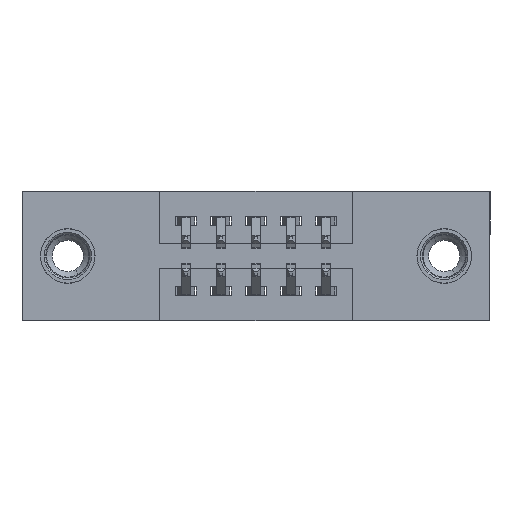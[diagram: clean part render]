
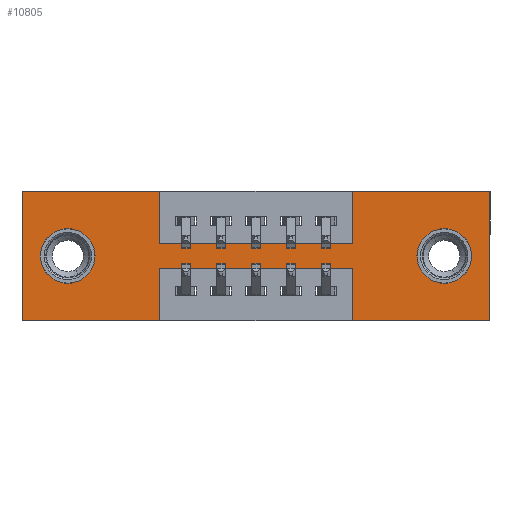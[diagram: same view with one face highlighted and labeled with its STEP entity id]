
A CAD part, front view. The second image highlights one B-rep face of the part: STEP entity #10805.
In plain terms, the highlighted planar face has unit normal (0, -1, 0).
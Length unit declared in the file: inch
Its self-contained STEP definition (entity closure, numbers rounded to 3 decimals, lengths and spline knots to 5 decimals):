
#29 = VERTEX_POINT ( 'NONE', #152 ) ;
#90 = LINE ( 'NONE', #10224, #9237 ) ;
#152 = CARTESIAN_POINT ( 'NONE',  ( 0.3925, 0., -0.37 ) ) ;
#196 = LINE ( 'NONE', #558, #7060 ) ;
#227 = DIRECTION ( 'NONE',  ( 0., -1., 0. ) ) ;
#324 = CARTESIAN_POINT ( 'NONE',  ( 0.9425, 0., -0.37 ) ) ;
#452 = DIRECTION ( 'NONE',  ( 0., 1., 0. ) ) ;
#520 = EDGE_LOOP ( 'NONE', ( #9153, #6924 ) ) ;
#558 = CARTESIAN_POINT ( 'NONE',  ( 0., 0., 0. ) ) ;
#603 = CARTESIAN_POINT ( 'NONE',  ( 0.13, 0., -0.107 ) ) ;
#827 = VERTEX_POINT ( 'NONE', #324 ) ;
#832 = EDGE_LOOP ( 'NONE', ( #2418, #1448 ) ) ;
#889 = CARTESIAN_POINT ( 'NONE',  ( 0.3925, 0., 0. ) ) ;
#953 = VERTEX_POINT ( 'NONE', #5917 ) ;
#1005 = AXIS2_PLACEMENT_3D ( 'NONE', #3215, #3204, #3176 ) ;
#1339 = CARTESIAN_POINT ( 'NONE',  ( 1.205, 0., -0.263 ) ) ;
#1391 = EDGE_CURVE ( 'NONE', #9028, #10332, #6580, .T. ) ;
#1403 = CARTESIAN_POINT ( 'NONE',  ( 0.9425, 0., -0.22 ) ) ;
#1415 = LINE ( 'NONE', #2271, #8147 ) ;
#1448 = ORIENTED_EDGE ( 'NONE', *, *, #3279, .T. ) ;
#1508 = ORIENTED_EDGE ( 'NONE', *, *, #8458, .F. ) ;
#1509 = DIRECTION ( 'NONE',  ( 1., 0., 0. ) ) ;
#1518 = ORIENTED_EDGE ( 'NONE', *, *, #10846, .F. ) ;
#1532 = VERTEX_POINT ( 'NONE', #1730 ) ;
#1537 = ORIENTED_EDGE ( 'NONE', *, *, #2017, .F. ) ;
#1550 = ORIENTED_EDGE ( 'NONE', *, *, #4668, .F. ) ;
#1585 = VECTOR ( 'NONE', #7772, 39.37008 ) ;
#1627 = EDGE_CURVE ( 'NONE', #7765, #827, #2035, .T. ) ;
#1730 = CARTESIAN_POINT ( 'NONE',  ( 0.9425, 0., -0.15 ) ) ;
#1786 = VERTEX_POINT ( 'NONE', #5215 ) ;
#1907 = EDGE_CURVE ( 'NONE', #4966, #5875, #4269, .T. ) ;
#2017 = EDGE_CURVE ( 'NONE', #3804, #7765, #5491, .T. ) ;
#2035 = LINE ( 'NONE', #3509, #6430 ) ;
#2183 = DIRECTION ( 'NONE',  ( 0., 0., 1. ) ) ;
#2238 = VECTOR ( 'NONE', #8586, 39.37008 ) ;
#2268 = CARTESIAN_POINT ( 'NONE',  ( 0.3925, 0., -0.22 ) ) ;
#2271 = CARTESIAN_POINT ( 'NONE',  ( 0.9425, 0., -0.37 ) ) ;
#2400 = EDGE_CURVE ( 'NONE', #10332, #29, #6279, .T. ) ;
#2418 = ORIENTED_EDGE ( 'NONE', *, *, #10934, .T. ) ;
#2457 = LINE ( 'NONE', #4250, #9087 ) ;
#2531 = EDGE_CURVE ( 'NONE', #4378, #1532, #5475, .T. ) ;
#2678 = CARTESIAN_POINT ( 'NONE',  ( 0.13, 0., -0.185 ) ) ;
#3044 = CARTESIAN_POINT ( 'NONE',  ( 0.9425, 0., 0. ) ) ;
#3176 = DIRECTION ( 'NONE',  ( 0., 0., 1. ) ) ;
#3204 = DIRECTION ( 'NONE',  ( 0., 1., 0. ) ) ;
#3215 = CARTESIAN_POINT ( 'NONE',  ( 0.13, 0., -0.185 ) ) ;
#3248 = LINE ( 'NONE', #9326, #9822 ) ;
#3279 = EDGE_CURVE ( 'NONE', #10318, #953, #9589, .T. ) ;
#3509 = CARTESIAN_POINT ( 'NONE',  ( 0., 0., -0.37 ) ) ;
#3572 = DIRECTION ( 'NONE',  ( 0., 0., 1. ) ) ;
#3727 = DIRECTION ( 'NONE',  ( 0., 0., -1. ) ) ;
#3750 = DIRECTION ( 'NONE',  ( 0., 1., 0. ) ) ;
#3784 = CARTESIAN_POINT ( 'NONE',  ( 1.205, 0., -0.185 ) ) ;
#3804 = VERTEX_POINT ( 'NONE', #10562 ) ;
#3896 = EDGE_CURVE ( 'NONE', #29, #6833, #3248, .T. ) ;
#3912 = CARTESIAN_POINT ( 'NONE',  ( 0., 0., -0.37 ) ) ;
#4129 = EDGE_CURVE ( 'NONE', #5875, #4966, #5434, .T. ) ;
#4250 = CARTESIAN_POINT ( 'NONE',  ( 0., 0., 0. ) ) ;
#4269 = CIRCLE ( 'NONE', #1005, 0.078 ) ;
#4378 = VERTEX_POINT ( 'NONE', #5546 ) ;
#4589 = LINE ( 'NONE', #7727, #2238 ) ;
#4656 = CARTESIAN_POINT ( 'NONE',  ( 0.13, 0., -0.263 ) ) ;
#4668 = EDGE_CURVE ( 'NONE', #1786, #3804, #4589, .T. ) ;
#4685 = ORIENTED_EDGE ( 'NONE', *, *, #9633, .F. ) ;
#4820 = CARTESIAN_POINT ( 'NONE',  ( 0., 0., -0.37 ) ) ;
#4946 = VECTOR ( 'NONE', #2183, 39.37008 ) ;
#4947 = DIRECTION ( 'NONE',  ( 0., 0., 1. ) ) ;
#4966 = VERTEX_POINT ( 'NONE', #4656 ) ;
#5127 = DIRECTION ( 'NONE',  ( 0., 0., -1. ) ) ;
#5215 = CARTESIAN_POINT ( 'NONE',  ( 0.9425, 0., 0. ) ) ;
#5327 = DIRECTION ( 'NONE',  ( -1., 0., 0. ) ) ;
#5373 = ORIENTED_EDGE ( 'NONE', *, *, #1391, .F. ) ;
#5434 = CIRCLE ( 'NONE', #10303, 0.078 ) ;
#5475 = LINE ( 'NONE', #7199, #9731 ) ;
#5491 = LINE ( 'NONE', #5619, #9745 ) ;
#5495 = FACE_BOUND ( 'NONE', #832, .T. ) ;
#5546 = CARTESIAN_POINT ( 'NONE',  ( 0.3925, 0., -0.15 ) ) ;
#5549 = DIRECTION ( 'NONE',  ( 0., 0., -1. ) ) ;
#5619 = CARTESIAN_POINT ( 'NONE',  ( 1.335, 0., 0. ) ) ;
#5656 = PLANE ( 'NONE',  #7951 ) ;
#5764 = FACE_BOUND ( 'NONE', #520, .T. ) ;
#5801 = ORIENTED_EDGE ( 'NONE', *, *, #3896, .F. ) ;
#5832 = CARTESIAN_POINT ( 'NONE',  ( 1.205, 0., -0.185 ) ) ;
#5875 = VERTEX_POINT ( 'NONE', #603 ) ;
#5917 = CARTESIAN_POINT ( 'NONE',  ( 1.205, 0., -0.107 ) ) ;
#5991 = CARTESIAN_POINT ( 'NONE',  ( 0.3925, 0., -0.37 ) ) ;
#6013 = ORIENTED_EDGE ( 'NONE', *, *, #2531, .F. ) ;
#6158 = CIRCLE ( 'NONE', #10194, 0.078 ) ;
#6216 = ORIENTED_EDGE ( 'NONE', *, *, #2400, .F. ) ;
#6279 = LINE ( 'NONE', #5991, #1585 ) ;
#6430 = VECTOR ( 'NONE', #5327, 39.37008 ) ;
#6432 = ORIENTED_EDGE ( 'NONE', *, *, #9747, .F. ) ;
#6515 = DIRECTION ( 'NONE',  ( 0., 0., -1. ) ) ;
#6580 = LINE ( 'NONE', #8602, #10785 ) ;
#6704 = DIRECTION ( 'NONE',  ( 0., 0., -1. ) ) ;
#6833 = VERTEX_POINT ( 'NONE', #4820 ) ;
#6924 = ORIENTED_EDGE ( 'NONE', *, *, #1907, .T. ) ;
#7060 = VECTOR ( 'NONE', #1509, 39.37008 ) ;
#7199 = CARTESIAN_POINT ( 'NONE',  ( 0.3925, 0., -0.15 ) ) ;
#7727 = CARTESIAN_POINT ( 'NONE',  ( 0., 0., 0. ) ) ;
#7765 = VERTEX_POINT ( 'NONE', #10062 ) ;
#7772 = DIRECTION ( 'NONE',  ( 0., 0., -1. ) ) ;
#7951 = AXIS2_PLACEMENT_3D ( 'NONE', #3912, #227, #6515 ) ;
#8147 = VECTOR ( 'NONE', #4947, 39.37008 ) ;
#8458 = EDGE_CURVE ( 'NONE', #6833, #10742, #2457, .T. ) ;
#8586 = DIRECTION ( 'NONE',  ( 1., 0., 0. ) ) ;
#8602 = CARTESIAN_POINT ( 'NONE',  ( 0.3925, 0., -0.22 ) ) ;
#8731 = DIRECTION ( 'NONE',  ( 0., 1., 0. ) ) ;
#9028 = VERTEX_POINT ( 'NONE', #1403 ) ;
#9087 = VECTOR ( 'NONE', #10974, 39.37008 ) ;
#9130 = ORIENTED_EDGE ( 'NONE', *, *, #10443, .F. ) ;
#9153 = ORIENTED_EDGE ( 'NONE', *, *, #4129, .T. ) ;
#9237 = VECTOR ( 'NONE', #5127, 39.37008 ) ;
#9326 = CARTESIAN_POINT ( 'NONE',  ( 0., 0., -0.37 ) ) ;
#9589 = CIRCLE ( 'NONE', #9659, 0.078 ) ;
#9633 = EDGE_CURVE ( 'NONE', #827, #9028, #1415, .T. ) ;
#9659 = AXIS2_PLACEMENT_3D ( 'NONE', #3784, #3750, #3727 ) ;
#9662 = DIRECTION ( 'NONE',  ( 1., 0., 0. ) ) ;
#9686 = DIRECTION ( 'NONE',  ( -1., 0., 0. ) ) ;
#9731 = VECTOR ( 'NONE', #9662, 39.37008 ) ;
#9745 = VECTOR ( 'NONE', #5549, 39.37008 ) ;
#9747 = EDGE_CURVE ( 'NONE', #10742, #10017, #196, .T. ) ;
#9749 = LINE ( 'NONE', #3044, #4946 ) ;
#9804 = CARTESIAN_POINT ( 'NONE',  ( 0., 0., 0. ) ) ;
#9822 = VECTOR ( 'NONE', #9686, 39.37008 ) ;
#9861 = EDGE_LOOP ( 'NONE', ( #6216, #5373, #4685, #11009, #1537, #1550, #1518, #6013, #9130, #6432, #1508, #5801 ) ) ;
#10017 = VERTEX_POINT ( 'NONE', #889 ) ;
#10023 = FACE_OUTER_BOUND ( 'NONE', #9861, .T. ) ;
#10062 = CARTESIAN_POINT ( 'NONE',  ( 1.335, 0., -0.37 ) ) ;
#10194 = AXIS2_PLACEMENT_3D ( 'NONE', #5832, #452, #6704 ) ;
#10224 = CARTESIAN_POINT ( 'NONE',  ( 0.3925, 0., 0. ) ) ;
#10303 = AXIS2_PLACEMENT_3D ( 'NONE', #2678, #8731, #3572 ) ;
#10318 = VERTEX_POINT ( 'NONE', #1339 ) ;
#10332 = VERTEX_POINT ( 'NONE', #2268 ) ;
#10443 = EDGE_CURVE ( 'NONE', #10017, #4378, #90, .T. ) ;
#10562 = CARTESIAN_POINT ( 'NONE',  ( 1.335, 0., 0. ) ) ;
#10742 = VERTEX_POINT ( 'NONE', #9804 ) ;
#10785 = VECTOR ( 'NONE', #11220, 39.37008 ) ;
#10805 = ADVANCED_FACE ( 'NONE', ( #5495, #5764, #10023 ), #5656, .T. ) ;
#10846 = EDGE_CURVE ( 'NONE', #1532, #1786, #9749, .T. ) ;
#10934 = EDGE_CURVE ( 'NONE', #953, #10318, #6158, .T. ) ;
#10974 = DIRECTION ( 'NONE',  ( 0., 0., 1. ) ) ;
#11009 = ORIENTED_EDGE ( 'NONE', *, *, #1627, .F. ) ;
#11220 = DIRECTION ( 'NONE',  ( -1., 0., 0. ) ) ;
